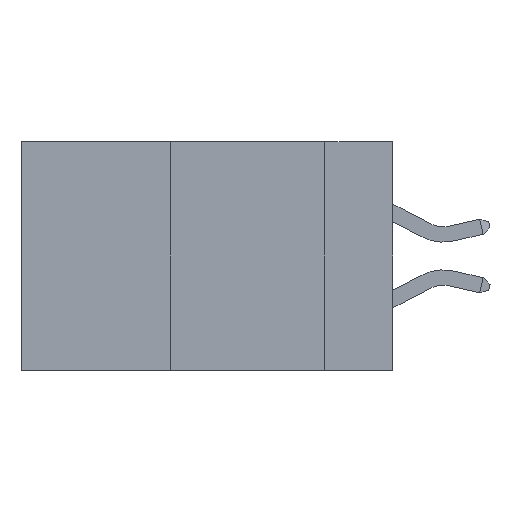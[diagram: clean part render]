
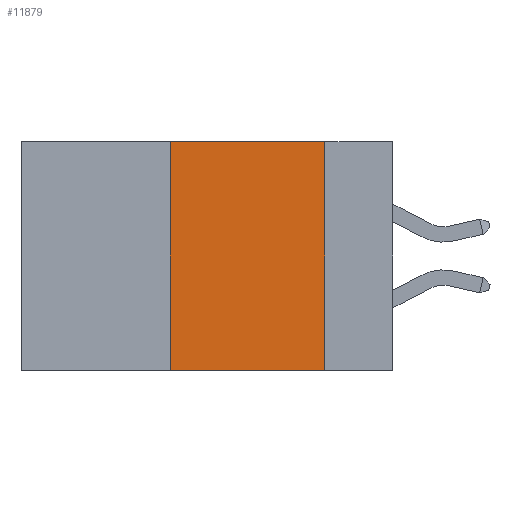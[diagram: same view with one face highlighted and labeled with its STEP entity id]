
A CAD part, left-side view. The second image highlights one B-rep face of the part: STEP entity #11879.
In plain terms, the highlighted planar face has unit normal (-1, 0, 0).
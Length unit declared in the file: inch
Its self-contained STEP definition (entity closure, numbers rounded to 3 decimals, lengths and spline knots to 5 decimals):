
#84 = FACE_OUTER_BOUND ( 'NONE', #2449, .T. ) ;
#2258 = DIRECTION ( 'NONE',  ( 1., 0., 0. ) ) ;
#2304 = EDGE_CURVE ( 'NONE', #17242, #8366, #21675, .T. ) ;
#2449 = EDGE_LOOP ( 'NONE', ( #11433, #16118, #16341, #11693 ) ) ;
#2567 = LINE ( 'NONE', #12255, #24477 ) ;
#4315 = EDGE_CURVE ( 'NONE', #12807, #22129, #20453, .T. ) ;
#4343 = PLANE ( 'NONE',  #22079 ) ;
#7586 = EDGE_CURVE ( 'NONE', #17242, #22129, #2567, .T. ) ;
#8155 = DIRECTION ( 'NONE',  ( 0., 0., -1. ) ) ;
#8366 = VERTEX_POINT ( 'NONE', #18765 ) ;
#8530 = VECTOR ( 'NONE', #14821, 39.37008 ) ;
#9728 = CARTESIAN_POINT ( 'NONE',  ( 0., 0.11, 0. ) ) ;
#10953 = LINE ( 'NONE', #18390, #8530 ) ;
#11433 = ORIENTED_EDGE ( 'NONE', *, *, #4315, .F. ) ;
#11693 = ORIENTED_EDGE ( 'NONE', *, *, #7586, .T. ) ;
#11879 = ADVANCED_FACE ( 'NONE', ( #84 ), #4343, .F. ) ;
#12255 = CARTESIAN_POINT ( 'NONE',  ( 0., 0.6, -0.37 ) ) ;
#12807 = VERTEX_POINT ( 'NONE', #24800 ) ;
#13829 = CARTESIAN_POINT ( 'NONE',  ( 0., 0.6, 0. ) ) ;
#14821 = DIRECTION ( 'NONE',  ( 0., -1., 0. ) ) ;
#15277 = VECTOR ( 'NONE', #21168, 39.37008 ) ;
#16118 = ORIENTED_EDGE ( 'NONE', *, *, #23690, .F. ) ;
#16341 = ORIENTED_EDGE ( 'NONE', *, *, #2304, .F. ) ;
#17242 = VERTEX_POINT ( 'NONE', #22069 ) ;
#18390 = CARTESIAN_POINT ( 'NONE',  ( 0., 0.6, 0. ) ) ;
#18765 = CARTESIAN_POINT ( 'NONE',  ( 0., 0.36, 0. ) ) ;
#20453 = LINE ( 'NONE', #9728, #15277 ) ;
#20559 = DIRECTION ( 'NONE',  ( 0., 0., 1. ) ) ;
#21168 = DIRECTION ( 'NONE',  ( 0., 0., -1. ) ) ;
#21171 = CARTESIAN_POINT ( 'NONE',  ( 0., 0.11, -0.37 ) ) ;
#21675 = LINE ( 'NONE', #22340, #23792 ) ;
#22069 = CARTESIAN_POINT ( 'NONE',  ( 0., 0.36, -0.37 ) ) ;
#22079 = AXIS2_PLACEMENT_3D ( 'NONE', #13829, #2258, #8155 ) ;
#22129 = VERTEX_POINT ( 'NONE', #21171 ) ;
#22209 = DIRECTION ( 'NONE',  ( 0., -1., 0. ) ) ;
#22340 = CARTESIAN_POINT ( 'NONE',  ( 0., 0.36, 0. ) ) ;
#23690 = EDGE_CURVE ( 'NONE', #8366, #12807, #10953, .T. ) ;
#23792 = VECTOR ( 'NONE', #20559, 39.37008 ) ;
#24477 = VECTOR ( 'NONE', #22209, 39.37008 ) ;
#24800 = CARTESIAN_POINT ( 'NONE',  ( 0., 0.11, 0. ) ) ;
